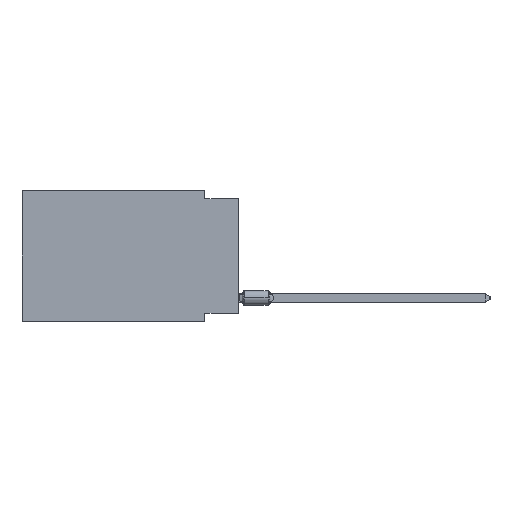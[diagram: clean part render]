
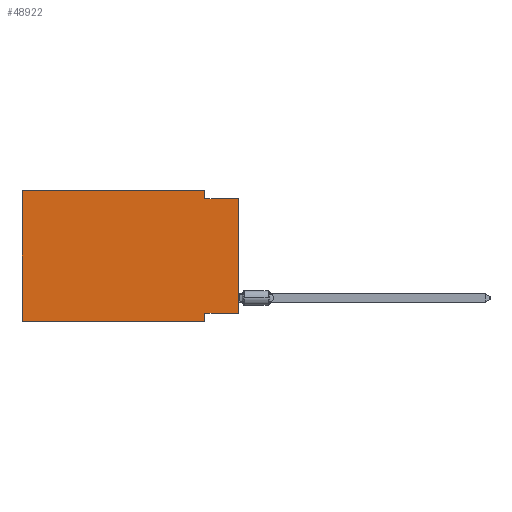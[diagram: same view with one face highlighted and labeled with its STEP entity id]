
A CAD part, left-side view. The second image highlights one B-rep face of the part: STEP entity #48922.
In plain terms, the highlighted planar face has unit normal (-1, 0, 0).
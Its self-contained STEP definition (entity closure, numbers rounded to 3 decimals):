
#1344 = CARTESIAN_POINT ( 'NONE',  ( 0., 2.54, 0. ) ) ;
#1551 = VECTOR ( 'NONE', #28604, 1000. ) ;
#2979 = CARTESIAN_POINT ( 'NONE',  ( 0., 0., -9.271 ) ) ;
#4976 = CARTESIAN_POINT ( 'NONE',  ( 0., 0., -0.635 ) ) ;
#5337 = DIRECTION ( 'NONE',  ( 0., 0., 1. ) ) ;
#5790 = EDGE_CURVE ( 'NONE', #59178, #28203, #23692, .T. ) ;
#6698 = CARTESIAN_POINT ( 'NONE',  ( 0., 2.54, -9.906 ) ) ;
#7067 = CARTESIAN_POINT ( 'NONE',  ( 0., 16.383, -9.906 ) ) ;
#8644 = VECTOR ( 'NONE', #5337, 1000. ) ;
#8723 = ORIENTED_EDGE ( 'NONE', *, *, #61228, .F. ) ;
#10512 = LINE ( 'NONE', #4976, #1551 ) ;
#12017 = AXIS2_PLACEMENT_3D ( 'NONE', #20394, #65462, #14860 ) ;
#12838 = VECTOR ( 'NONE', #34789, 1000. ) ;
#14499 = PLANE ( 'NONE',  #12017 ) ;
#14860 = DIRECTION ( 'NONE',  ( 0., 0., -1. ) ) ;
#15023 = ORIENTED_EDGE ( 'NONE', *, *, #61250, .T. ) ;
#15136 = DIRECTION ( 'NONE',  ( 0., 1., 0. ) ) ;
#15497 = LINE ( 'NONE', #2979, #18604 ) ;
#16819 = DIRECTION ( 'NONE',  ( 0., 0., -1. ) ) ;
#17924 = CARTESIAN_POINT ( 'NONE',  ( 0., 16.383, -9.906 ) ) ;
#18293 = EDGE_CURVE ( 'NONE', #37933, #28203, #62842, .T. ) ;
#18604 = VECTOR ( 'NONE', #15136, 1000. ) ;
#20394 = CARTESIAN_POINT ( 'NONE',  ( 0., 16.383, 0. ) ) ;
#21131 = EDGE_LOOP ( 'NONE', ( #15023, #8723, #66237, #24390, #69784, #57557, #40244, #70964 ) ) ;
#23692 = LINE ( 'NONE', #63207, #46542 ) ;
#24128 = LINE ( 'NONE', #34873, #34445 ) ;
#24390 = ORIENTED_EDGE ( 'NONE', *, *, #48742, .F. ) ;
#24508 = DIRECTION ( 'NONE',  ( 0., -1., 0. ) ) ;
#25442 = CARTESIAN_POINT ( 'NONE',  ( 0., 2.54, -0.635 ) ) ;
#28203 = VERTEX_POINT ( 'NONE', #6698 ) ;
#28457 = VERTEX_POINT ( 'NONE', #72001 ) ;
#28604 = DIRECTION ( 'NONE',  ( 0., -1., 0. ) ) ;
#33063 = CARTESIAN_POINT ( 'NONE',  ( 0., 0., 0. ) ) ;
#33469 = EDGE_CURVE ( 'NONE', #56255, #62383, #39747, .T. ) ;
#34210 = CARTESIAN_POINT ( 'NONE',  ( 0., 2.54, 0. ) ) ;
#34445 = VECTOR ( 'NONE', #24508, 1000. ) ;
#34789 = DIRECTION ( 'NONE',  ( 0., -1., 0. ) ) ;
#34873 = CARTESIAN_POINT ( 'NONE',  ( 0., 16.383, 0. ) ) ;
#35490 = VERTEX_POINT ( 'NONE', #62453 ) ;
#35518 = VERTEX_POINT ( 'NONE', #51378 ) ;
#35780 = VECTOR ( 'NONE', #16819, 1000. ) ;
#37840 = EDGE_CURVE ( 'NONE', #37933, #35490, #61543, .T. ) ;
#37933 = VERTEX_POINT ( 'NONE', #17924 ) ;
#39747 = LINE ( 'NONE', #34210, #35780 ) ;
#40244 = ORIENTED_EDGE ( 'NONE', *, *, #5790, .F. ) ;
#46542 = VECTOR ( 'NONE', #50305, 1000. ) ;
#48742 = EDGE_CURVE ( 'NONE', #35490, #56255, #24128, .T. ) ;
#48922 = ADVANCED_FACE ( 'NONE', ( #71001 ), #14499, .F. ) ;
#50305 = DIRECTION ( 'NONE',  ( 0., 0., -1. ) ) ;
#51378 = CARTESIAN_POINT ( 'NONE',  ( 0., 0., -9.271 ) ) ;
#53848 = VECTOR ( 'NONE', #63365, 1000. ) ;
#56255 = VERTEX_POINT ( 'NONE', #1344 ) ;
#57557 = ORIENTED_EDGE ( 'NONE', *, *, #18293, .T. ) ;
#57909 = CARTESIAN_POINT ( 'NONE',  ( 0., 2.54, -9.271 ) ) ;
#59178 = VERTEX_POINT ( 'NONE', #57909 ) ;
#61228 = EDGE_CURVE ( 'NONE', #62383, #28457, #10512, .T. ) ;
#61250 = EDGE_CURVE ( 'NONE', #35518, #28457, #72195, .T. ) ;
#61543 = LINE ( 'NONE', #68181, #53848 ) ;
#62383 = VERTEX_POINT ( 'NONE', #25442 ) ;
#62453 = CARTESIAN_POINT ( 'NONE',  ( 0., 16.383, 0. ) ) ;
#62842 = LINE ( 'NONE', #7067, #12838 ) ;
#63207 = CARTESIAN_POINT ( 'NONE',  ( 0., 2.54, -9.906 ) ) ;
#63365 = DIRECTION ( 'NONE',  ( 0., 0., 1. ) ) ;
#64699 = EDGE_CURVE ( 'NONE', #35518, #59178, #15497, .T. ) ;
#65462 = DIRECTION ( 'NONE',  ( 1., 0., 0. ) ) ;
#66237 = ORIENTED_EDGE ( 'NONE', *, *, #33469, .F. ) ;
#68181 = CARTESIAN_POINT ( 'NONE',  ( 0., 16.383, 0. ) ) ;
#69784 = ORIENTED_EDGE ( 'NONE', *, *, #37840, .F. ) ;
#70964 = ORIENTED_EDGE ( 'NONE', *, *, #64699, .F. ) ;
#71001 = FACE_OUTER_BOUND ( 'NONE', #21131, .T. ) ;
#72001 = CARTESIAN_POINT ( 'NONE',  ( 0., 0., -0.635 ) ) ;
#72195 = LINE ( 'NONE', #33063, #8644 ) ;
